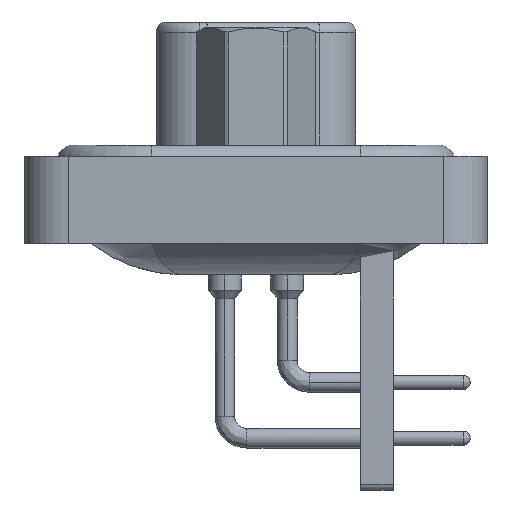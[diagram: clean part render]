
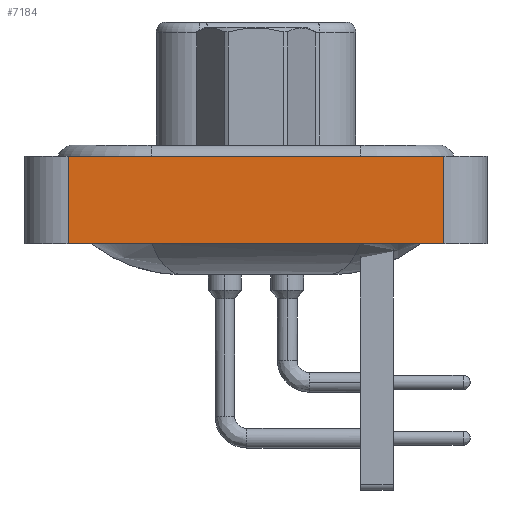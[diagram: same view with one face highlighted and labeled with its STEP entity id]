
A CAD part, left-side view. The second image highlights one B-rep face of the part: STEP entity #7184.
In plain terms, the highlighted planar face has unit normal (-1, 0, 0).
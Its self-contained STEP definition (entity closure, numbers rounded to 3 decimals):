
#2163 = AXIS2_PLACEMENT_3D ( 'NONE', #30613, #9608, #17191 ) ;
#4717 = CARTESIAN_POINT ( 'NONE',  ( -7.35, -8.55, -3.6 ) ) ;
#5700 = VERTEX_POINT ( 'NONE', #17090 ) ;
#7184 = ADVANCED_FACE ( 'NONE', ( #21855 ), #25085, .T. ) ;
#7279 = EDGE_LOOP ( 'NONE', ( #30307, #23564, #10547, #8224 ) ) ;
#8146 = VECTOR ( 'NONE', #25150, 1000. ) ;
#8224 = ORIENTED_EDGE ( 'NONE', *, *, #31327, .T. ) ;
#9600 = DIRECTION ( 'NONE',  ( 0., -1., 0. ) ) ;
#9608 = DIRECTION ( 'NONE',  ( -1., 0., 0. ) ) ;
#10111 = VECTOR ( 'NONE', #30679, 1000. ) ;
#10221 = LINE ( 'NONE', #30097, #8146 ) ;
#10260 = VECTOR ( 'NONE', #9600, 1000. ) ;
#10547 = ORIENTED_EDGE ( 'NONE', *, *, #31824, .F. ) ;
#11109 = EDGE_CURVE ( 'NONE', #5700, #12866, #27368, .T. ) ;
#12219 = CARTESIAN_POINT ( 'NONE',  ( -7.35, 8.55, 0.4 ) ) ;
#12447 = CARTESIAN_POINT ( 'NONE',  ( -7.35, 8.55, -3.6 ) ) ;
#12866 = VERTEX_POINT ( 'NONE', #20589 ) ;
#15646 = VERTEX_POINT ( 'NONE', #12447 ) ;
#17090 = CARTESIAN_POINT ( 'NONE',  ( -7.35, -8.55, -3.6 ) ) ;
#17191 = DIRECTION ( 'NONE',  ( 0., 0., 1. ) ) ;
#17765 = VECTOR ( 'NONE', #26160, 1000. ) ;
#20589 = CARTESIAN_POINT ( 'NONE',  ( -7.35, -8.55, 0.4 ) ) ;
#21751 = LINE ( 'NONE', #25308, #10260 ) ;
#21855 = FACE_OUTER_BOUND ( 'NONE', #7279, .T. ) ;
#23564 = ORIENTED_EDGE ( 'NONE', *, *, #27982, .F. ) ;
#24711 = LINE ( 'NONE', #26053, #17765 ) ;
#25085 = PLANE ( 'NONE',  #2163 ) ;
#25150 = DIRECTION ( 'NONE',  ( 0., 0., 1. ) ) ;
#25308 = CARTESIAN_POINT ( 'NONE',  ( -7.35, -8.55, -3.6 ) ) ;
#25802 = VERTEX_POINT ( 'NONE', #12219 ) ;
#26053 = CARTESIAN_POINT ( 'NONE',  ( -7.35, -8.55, 0.4 ) ) ;
#26160 = DIRECTION ( 'NONE',  ( 0., -1., 0. ) ) ;
#27368 = LINE ( 'NONE', #4717, #10111 ) ;
#27982 = EDGE_CURVE ( 'NONE', #25802, #12866, #24711, .T. ) ;
#30097 = CARTESIAN_POINT ( 'NONE',  ( -7.35, 8.55, -3.6 ) ) ;
#30307 = ORIENTED_EDGE ( 'NONE', *, *, #11109, .T. ) ;
#30613 = CARTESIAN_POINT ( 'NONE',  ( -7.35, -8.55, -3.6 ) ) ;
#30679 = DIRECTION ( 'NONE',  ( 0., 0., 1. ) ) ;
#31327 = EDGE_CURVE ( 'NONE', #15646, #5700, #21751, .T. ) ;
#31824 = EDGE_CURVE ( 'NONE', #15646, #25802, #10221, .T. ) ;
